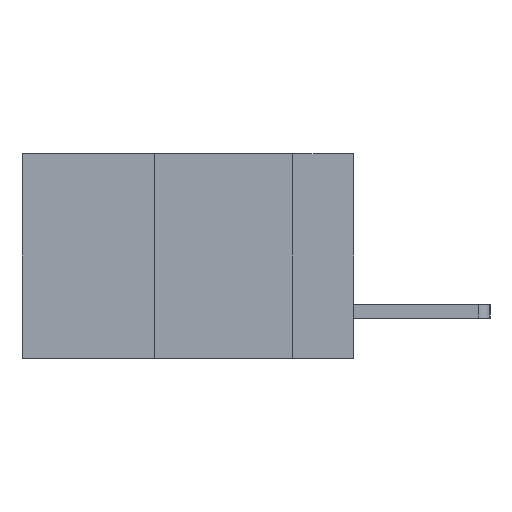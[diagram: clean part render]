
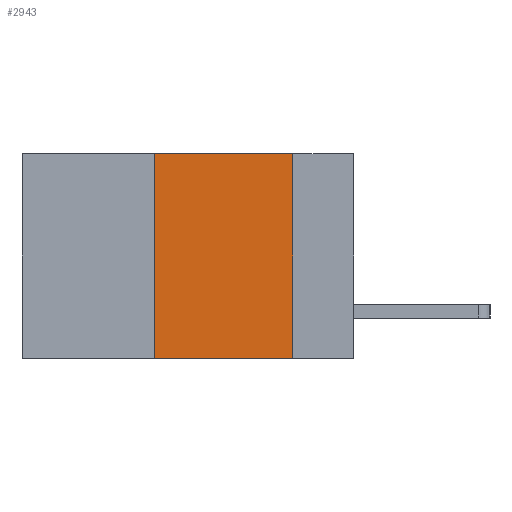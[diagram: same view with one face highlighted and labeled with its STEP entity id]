
A CAD part, left-side view. The second image highlights one B-rep face of the part: STEP entity #2943.
In plain terms, the highlighted planar face has unit normal (-1, 0, 0).
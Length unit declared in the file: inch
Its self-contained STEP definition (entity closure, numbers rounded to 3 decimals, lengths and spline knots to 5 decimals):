
#628 = LINE ( 'NONE', #6259, #12110 ) ;
#940 = LINE ( 'NONE', #12985, #2391 ) ;
#1053 = CARTESIAN_POINT ( 'NONE',  ( 0., 0.6, 0. ) ) ;
#1088 = CARTESIAN_POINT ( 'NONE',  ( 0., 0.11, 0. ) ) ;
#1518 = ORIENTED_EDGE ( 'NONE', *, *, #7897, .F. ) ;
#1986 = VERTEX_POINT ( 'NONE', #9996 ) ;
#2146 = PLANE ( 'NONE',  #12028 ) ;
#2171 = VECTOR ( 'NONE', #11063, 39.37008 ) ;
#2298 = VECTOR ( 'NONE', #2928, 39.37008 ) ;
#2391 = VECTOR ( 'NONE', #7375, 39.37008 ) ;
#2833 = EDGE_CURVE ( 'NONE', #13344, #5179, #3147, .T. ) ;
#2928 = DIRECTION ( 'NONE',  ( 0., 0., -1. ) ) ;
#2943 = ADVANCED_FACE ( 'NONE', ( #8936 ), #2146, .F. ) ;
#3147 = LINE ( 'NONE', #5379, #2298 ) ;
#4685 = VERTEX_POINT ( 'NONE', #6042 ) ;
#5179 = VERTEX_POINT ( 'NONE', #13005 ) ;
#5379 = CARTESIAN_POINT ( 'NONE',  ( 0., 0.11, 0. ) ) ;
#5446 = DIRECTION ( 'NONE',  ( 0., 0., -1. ) ) ;
#6042 = CARTESIAN_POINT ( 'NONE',  ( 0., 0.36, -0.37 ) ) ;
#6259 = CARTESIAN_POINT ( 'NONE',  ( 0., 0.6, 0. ) ) ;
#7375 = DIRECTION ( 'NONE',  ( 0., -1., 0. ) ) ;
#7897 = EDGE_CURVE ( 'NONE', #1986, #13344, #628, .T. ) ;
#8458 = ORIENTED_EDGE ( 'NONE', *, *, #2833, .F. ) ;
#8936 = FACE_OUTER_BOUND ( 'NONE', #11762, .T. ) ;
#9669 = DIRECTION ( 'NONE',  ( 0., -1., 0. ) ) ;
#9843 = ORIENTED_EDGE ( 'NONE', *, *, #10095, .T. ) ;
#9996 = CARTESIAN_POINT ( 'NONE',  ( 0., 0.36, 0. ) ) ;
#10095 = EDGE_CURVE ( 'NONE', #4685, #5179, #940, .T. ) ;
#10692 = EDGE_CURVE ( 'NONE', #4685, #1986, #13547, .T. ) ;
#11063 = DIRECTION ( 'NONE',  ( 0., 0., 1. ) ) ;
#11762 = EDGE_LOOP ( 'NONE', ( #8458, #1518, #11854, #9843 ) ) ;
#11854 = ORIENTED_EDGE ( 'NONE', *, *, #10692, .F. ) ;
#12028 = AXIS2_PLACEMENT_3D ( 'NONE', #1053, #13376, #5446 ) ;
#12110 = VECTOR ( 'NONE', #9669, 39.37008 ) ;
#12401 = CARTESIAN_POINT ( 'NONE',  ( 0., 0.36, 0. ) ) ;
#12985 = CARTESIAN_POINT ( 'NONE',  ( 0., 0.6, -0.37 ) ) ;
#13005 = CARTESIAN_POINT ( 'NONE',  ( 0., 0.11, -0.37 ) ) ;
#13344 = VERTEX_POINT ( 'NONE', #1088 ) ;
#13376 = DIRECTION ( 'NONE',  ( 1., 0., 0. ) ) ;
#13547 = LINE ( 'NONE', #12401, #2171 ) ;
